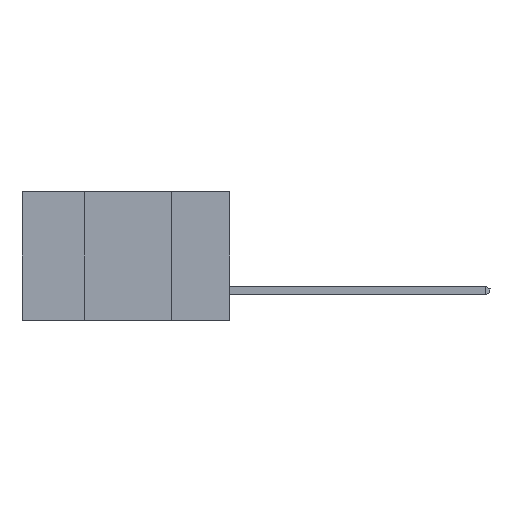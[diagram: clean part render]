
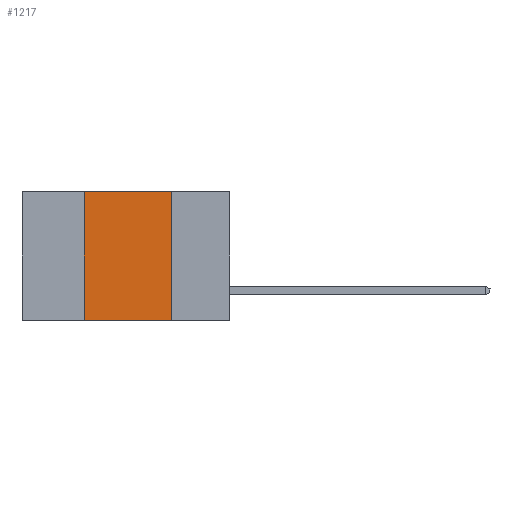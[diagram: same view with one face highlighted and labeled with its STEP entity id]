
A CAD part, left-side view. The second image highlights one B-rep face of the part: STEP entity #1217.
In plain terms, the highlighted planar face has unit normal (-1, 0, 0).
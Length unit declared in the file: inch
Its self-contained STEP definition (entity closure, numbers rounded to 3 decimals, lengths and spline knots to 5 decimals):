
#875 = VERTEX_POINT ( 'NONE', #19823 ) ;
#1141 = VECTOR ( 'NONE', #3421, 39.37008 ) ;
#1217 = ADVANCED_FACE ( 'NONE', ( #2444 ), #13412, .F. ) ;
#1498 = VECTOR ( 'NONE', #11844, 39.37008 ) ;
#2182 = ORIENTED_EDGE ( 'NONE', *, *, #23719, .F. ) ;
#2440 = VERTEX_POINT ( 'NONE', #12552 ) ;
#2444 = FACE_OUTER_BOUND ( 'NONE', #4437, .T. ) ;
#2698 = LINE ( 'NONE', #4768, #1498 ) ;
#3200 = AXIS2_PLACEMENT_3D ( 'NONE', #3283, #10711, #21980 ) ;
#3283 = CARTESIAN_POINT ( 'NONE',  ( 0., 0.6, 0. ) ) ;
#3421 = DIRECTION ( 'NONE',  ( 0., -1., 0. ) ) ;
#3552 = VECTOR ( 'NONE', #17871, 39.37008 ) ;
#4256 = LINE ( 'NONE', #15520, #17444 ) ;
#4437 = EDGE_LOOP ( 'NONE', ( #2182, #13470, #9917, #22645 ) ) ;
#4768 = CARTESIAN_POINT ( 'NONE',  ( 0., 0.42, -0.37 ) ) ;
#4787 = LINE ( 'NONE', #12599, #3552 ) ;
#9154 = EDGE_CURVE ( 'NONE', #875, #11997, #20273, .T. ) ;
#9917 = ORIENTED_EDGE ( 'NONE', *, *, #12699, .F. ) ;
#10711 = DIRECTION ( 'NONE',  ( 1., 0., 0. ) ) ;
#11844 = DIRECTION ( 'NONE',  ( 0., 0., 1. ) ) ;
#11997 = VERTEX_POINT ( 'NONE', #22423 ) ;
#12552 = CARTESIAN_POINT ( 'NONE',  ( 0., 0.42, 0. ) ) ;
#12599 = CARTESIAN_POINT ( 'NONE',  ( 0., 0.17, -0.37 ) ) ;
#12678 = CARTESIAN_POINT ( 'NONE',  ( 0., 0.6, -0.37 ) ) ;
#12699 = EDGE_CURVE ( 'NONE', #875, #2440, #2698, .T. ) ;
#13412 = PLANE ( 'NONE',  #3200 ) ;
#13470 = ORIENTED_EDGE ( 'NONE', *, *, #16176, .F. ) ;
#15520 = CARTESIAN_POINT ( 'NONE',  ( 0., 0.6, 0. ) ) ;
#16176 = EDGE_CURVE ( 'NONE', #2440, #20294, #4256, .T. ) ;
#17444 = VECTOR ( 'NONE', #21482, 39.37008 ) ;
#17871 = DIRECTION ( 'NONE',  ( 0., 0., -1. ) ) ;
#19823 = CARTESIAN_POINT ( 'NONE',  ( 0., 0.42, -0.37 ) ) ;
#20238 = CARTESIAN_POINT ( 'NONE',  ( 0., 0.17, 0. ) ) ;
#20273 = LINE ( 'NONE', #12678, #1141 ) ;
#20294 = VERTEX_POINT ( 'NONE', #20238 ) ;
#21482 = DIRECTION ( 'NONE',  ( 0., -1., 0. ) ) ;
#21980 = DIRECTION ( 'NONE',  ( 0., 0., -1. ) ) ;
#22423 = CARTESIAN_POINT ( 'NONE',  ( 0., 0.17, -0.37 ) ) ;
#22645 = ORIENTED_EDGE ( 'NONE', *, *, #9154, .T. ) ;
#23719 = EDGE_CURVE ( 'NONE', #20294, #11997, #4787, .T. ) ;
